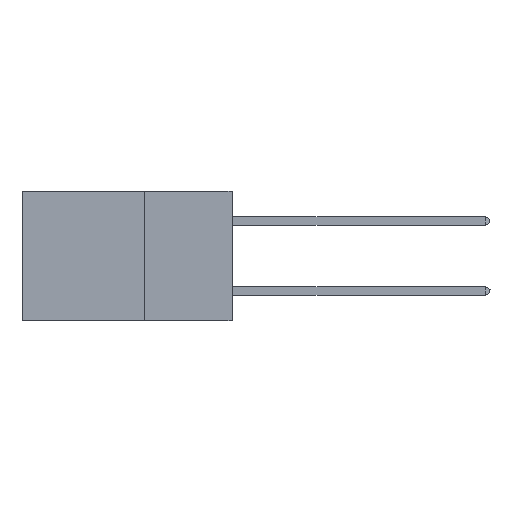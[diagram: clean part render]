
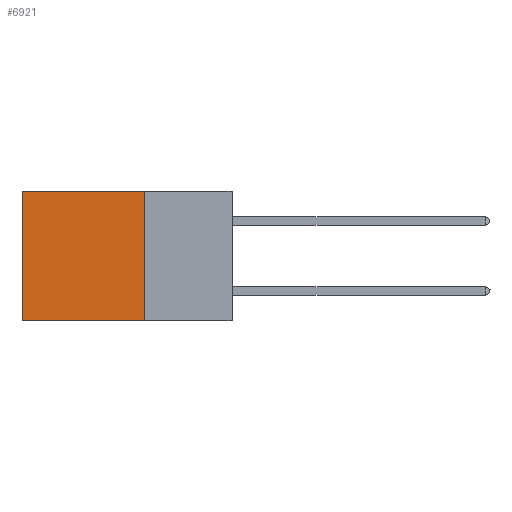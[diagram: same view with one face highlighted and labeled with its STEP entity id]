
A CAD part, left-side view. The second image highlights one B-rep face of the part: STEP entity #6921.
In plain terms, the highlighted planar face has unit normal (-1, 0, 0).
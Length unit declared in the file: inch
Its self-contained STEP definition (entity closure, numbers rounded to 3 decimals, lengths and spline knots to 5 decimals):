
#38 = CARTESIAN_POINT ( 'NONE',  ( 0.2875, 0.25, 0. ) ) ;
#2092 = VECTOR ( 'NONE', #3429, 39.37008 ) ;
#2257 = LINE ( 'NONE', #38, #32209 ) ;
#3429 = DIRECTION ( 'NONE',  ( 0., 0., -1. ) ) ;
#3574 = PLANE ( 'NONE',  #37786 ) ;
#4636 = CARTESIAN_POINT ( 'NONE',  ( 0.2875, 0.6, 0. ) ) ;
#5431 = CARTESIAN_POINT ( 'NONE',  ( 0.2875, 0.25, 0. ) ) ;
#6238 = DIRECTION ( 'NONE',  ( 0., 0., -1. ) ) ;
#6921 = ADVANCED_FACE ( 'NONE', ( #12737 ), #3574, .F. ) ;
#7002 = ORIENTED_EDGE ( 'NONE', *, *, #24439, .T. ) ;
#8022 = EDGE_CURVE ( 'NONE', #10518, #30933, #2257, .T. ) ;
#9844 = EDGE_CURVE ( 'NONE', #30933, #10769, #33762, .T. ) ;
#10518 = VERTEX_POINT ( 'NONE', #13767 ) ;
#10769 = VERTEX_POINT ( 'NONE', #39173 ) ;
#12173 = EDGE_LOOP ( 'NONE', ( #32153, #33655, #17028, #7002 ) ) ;
#12737 = FACE_OUTER_BOUND ( 'NONE', #12173, .T. ) ;
#12899 = VERTEX_POINT ( 'NONE', #4636 ) ;
#13767 = CARTESIAN_POINT ( 'NONE',  ( 0.2875, 0.25, 0. ) ) ;
#17026 = DIRECTION ( 'NONE',  ( 0., 1., 0. ) ) ;
#17028 = ORIENTED_EDGE ( 'NONE', *, *, #8022, .F. ) ;
#19159 = LINE ( 'NONE', #24933, #2092 ) ;
#20327 = EDGE_CURVE ( 'NONE', #12899, #10769, #19159, .T. ) ;
#22551 = DIRECTION ( 'NONE',  ( 0., 0., -1. ) ) ;
#23698 = VECTOR ( 'NONE', #32852, 39.37008 ) ;
#24439 = EDGE_CURVE ( 'NONE', #10518, #12899, #31802, .T. ) ;
#24933 = CARTESIAN_POINT ( 'NONE',  ( 0.2875, 0.6, 0. ) ) ;
#30933 = VERTEX_POINT ( 'NONE', #35997 ) ;
#31802 = LINE ( 'NONE', #5431, #23698 ) ;
#32153 = ORIENTED_EDGE ( 'NONE', *, *, #20327, .T. ) ;
#32209 = VECTOR ( 'NONE', #6238, 39.37008 ) ;
#32852 = DIRECTION ( 'NONE',  ( 0., 1., 0. ) ) ;
#33655 = ORIENTED_EDGE ( 'NONE', *, *, #9844, .F. ) ;
#33762 = LINE ( 'NONE', #38448, #34250 ) ;
#34250 = VECTOR ( 'NONE', #17026, 39.37008 ) ;
#34943 = CARTESIAN_POINT ( 'NONE',  ( 0.2875, 0.25, 0. ) ) ;
#35997 = CARTESIAN_POINT ( 'NONE',  ( 0.2875, 0.25, -0.37 ) ) ;
#37786 = AXIS2_PLACEMENT_3D ( 'NONE', #34943, #38134, #22551 ) ;
#38134 = DIRECTION ( 'NONE',  ( 1., 0., 0. ) ) ;
#38448 = CARTESIAN_POINT ( 'NONE',  ( 0.2875, 0.25, -0.37 ) ) ;
#39173 = CARTESIAN_POINT ( 'NONE',  ( 0.2875, 0.6, -0.37 ) ) ;
